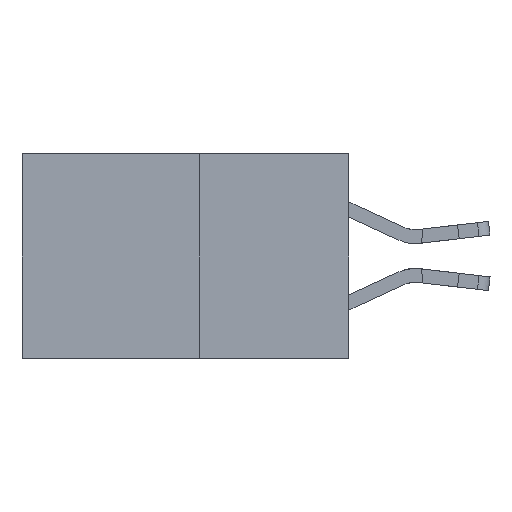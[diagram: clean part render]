
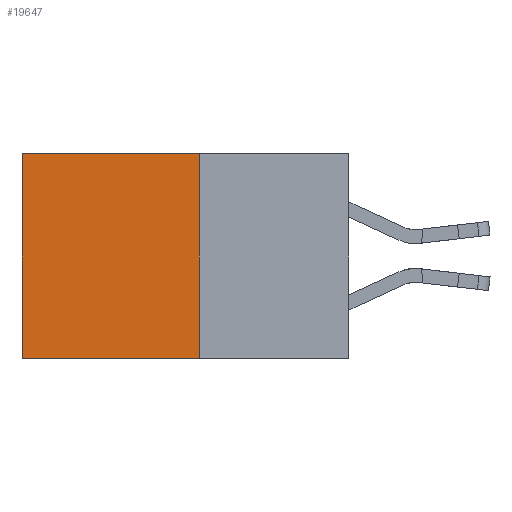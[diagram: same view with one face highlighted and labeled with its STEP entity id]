
A CAD part, left-side view. The second image highlights one B-rep face of the part: STEP entity #19647.
In plain terms, the highlighted planar face has unit normal (-1, 0, 0).
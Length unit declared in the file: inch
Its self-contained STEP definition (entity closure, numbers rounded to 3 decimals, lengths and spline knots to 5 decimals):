
#448 = ORIENTED_EDGE ( 'NONE', *, *, #3463, .F. ) ;
#526 = DIRECTION ( 'NONE',  ( 0., 0., -1. ) ) ;
#1230 = CARTESIAN_POINT ( 'NONE',  ( 0.277, 0.27, 0. ) ) ;
#1296 = EDGE_CURVE ( 'NONE', #4114, #19936, #8580, .T. ) ;
#1897 = ORIENTED_EDGE ( 'NONE', *, *, #1296, .T. ) ;
#2802 = DIRECTION ( 'NONE',  ( 0., 1., 0. ) ) ;
#3463 = EDGE_CURVE ( 'NONE', #3784, #20282, #11914, .T. ) ;
#3784 = VERTEX_POINT ( 'NONE', #16551 ) ;
#4114 = VERTEX_POINT ( 'NONE', #1230 ) ;
#4177 = EDGE_CURVE ( 'NONE', #19936, #20282, #23298, .T. ) ;
#4665 = VECTOR ( 'NONE', #2802, 39.37008 ) ;
#5081 = LINE ( 'NONE', #26420, #16966 ) ;
#5959 = VECTOR ( 'NONE', #25481, 39.37008 ) ;
#6199 = EDGE_CURVE ( 'NONE', #4114, #3784, #5081, .T. ) ;
#8580 = LINE ( 'NONE', #12573, #4665 ) ;
#9550 = CARTESIAN_POINT ( 'NONE',  ( 0.277, 0.27, -0.37 ) ) ;
#10978 = AXIS2_PLACEMENT_3D ( 'NONE', #9550, #14127, #526 ) ;
#11647 = CARTESIAN_POINT ( 'NONE',  ( 0.277, 0.59, -0.37 ) ) ;
#11914 = LINE ( 'NONE', #25667, #5959 ) ;
#12534 = ORIENTED_EDGE ( 'NONE', *, *, #6199, .F. ) ;
#12573 = CARTESIAN_POINT ( 'NONE',  ( 0.277, 0.27, 0. ) ) ;
#14127 = DIRECTION ( 'NONE',  ( 1., 0., 0. ) ) ;
#16551 = CARTESIAN_POINT ( 'NONE',  ( 0.277, 0.27, -0.37 ) ) ;
#16966 = VECTOR ( 'NONE', #26323, 39.37008 ) ;
#17419 = VECTOR ( 'NONE', #18865, 39.37008 ) ;
#18669 = FACE_OUTER_BOUND ( 'NONE', #21071, .T. ) ;
#18865 = DIRECTION ( 'NONE',  ( 0., 0., -1. ) ) ;
#19647 = ADVANCED_FACE ( 'NONE', ( #18669 ), #22888, .F. ) ;
#19936 = VERTEX_POINT ( 'NONE', #28067 ) ;
#20282 = VERTEX_POINT ( 'NONE', #11647 ) ;
#21071 = EDGE_LOOP ( 'NONE', ( #27367, #448, #12534, #1897 ) ) ;
#22888 = PLANE ( 'NONE',  #10978 ) ;
#23298 = LINE ( 'NONE', #24573, #17419 ) ;
#24573 = CARTESIAN_POINT ( 'NONE',  ( 0.277, 0.59, -0.37 ) ) ;
#25481 = DIRECTION ( 'NONE',  ( 0., 1., 0. ) ) ;
#25667 = CARTESIAN_POINT ( 'NONE',  ( 0.277, 0.27, -0.37 ) ) ;
#26323 = DIRECTION ( 'NONE',  ( 0., 0., -1. ) ) ;
#26420 = CARTESIAN_POINT ( 'NONE',  ( 0.277, 0.27, -0.37 ) ) ;
#27367 = ORIENTED_EDGE ( 'NONE', *, *, #4177, .T. ) ;
#28067 = CARTESIAN_POINT ( 'NONE',  ( 0.277, 0.59, 0. ) ) ;
